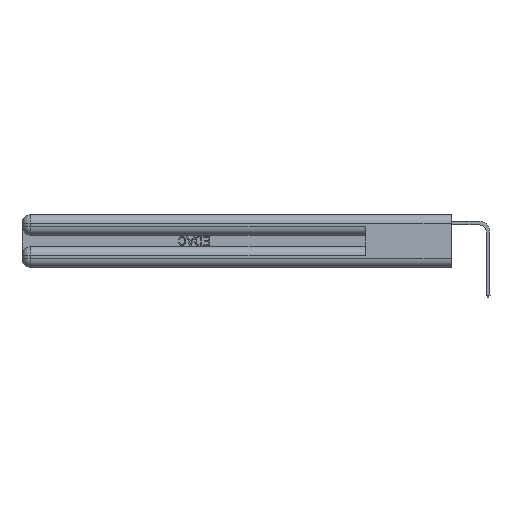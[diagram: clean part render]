
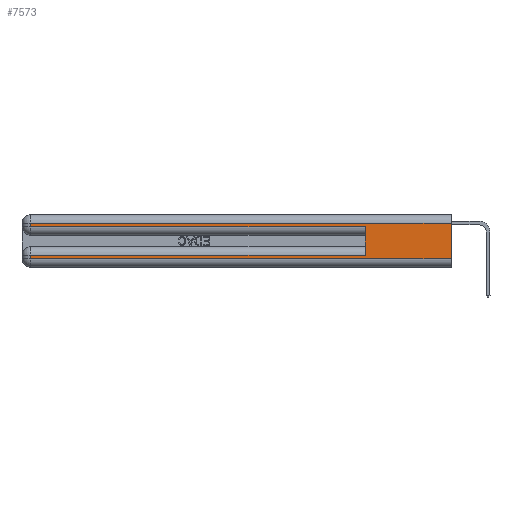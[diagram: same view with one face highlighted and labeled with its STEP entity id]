
A CAD part, left-side view. The second image highlights one B-rep face of the part: STEP entity #7573.
In plain terms, the highlighted planar face has unit normal (-1, 0, 0).
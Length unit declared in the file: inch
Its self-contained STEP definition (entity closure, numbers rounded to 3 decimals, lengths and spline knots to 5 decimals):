
#15 = VERTEX_POINT ( 'NONE', #14612 ) ;
#119 = CARTESIAN_POINT ( 'NONE',  ( 0., 0., 0.31 ) ) ;
#379 = VECTOR ( 'NONE', #6534, 39.37008 ) ;
#1182 = EDGE_CURVE ( 'NONE', #17346, #2728, #1530, .T. ) ;
#1530 = LINE ( 'NONE', #23896, #21152 ) ;
#1609 = LINE ( 'NONE', #19581, #3308 ) ;
#1701 = CARTESIAN_POINT ( 'NONE',  ( 0., 0.6, 0.285 ) ) ;
#2008 = LINE ( 'NONE', #19993, #13418 ) ;
#2155 = DIRECTION ( 'NONE',  ( 0., 1., 0. ) ) ;
#2191 = CARTESIAN_POINT ( 'NONE',  ( 0., 0., 0.37 ) ) ;
#2675 = CARTESIAN_POINT ( 'NONE',  ( 0., 2.94, 0.31 ) ) ;
#2728 = VERTEX_POINT ( 'NONE', #1701 ) ;
#3160 = ORIENTED_EDGE ( 'NONE', *, *, #20132, .T. ) ;
#3249 = CARTESIAN_POINT ( 'NONE',  ( 0., 0., 0.37 ) ) ;
#3308 = VECTOR ( 'NONE', #12978, 39.37008 ) ;
#3700 = CARTESIAN_POINT ( 'NONE',  ( 0., 0., 0.31 ) ) ;
#3762 = VERTEX_POINT ( 'NONE', #2675 ) ;
#5946 = VECTOR ( 'NONE', #15485, 39.37008 ) ;
#6268 = EDGE_CURVE ( 'NONE', #24456, #2728, #8498, .T. ) ;
#6534 = DIRECTION ( 'NONE',  ( 0., -1., 0. ) ) ;
#7437 = ORIENTED_EDGE ( 'NONE', *, *, #15135, .T. ) ;
#7573 = ADVANCED_FACE ( 'NONE', ( #27654 ), #14335, .F. ) ;
#8056 = DIRECTION ( 'NONE',  ( 0., -1., 0. ) ) ;
#8498 = LINE ( 'NONE', #26365, #9792 ) ;
#9051 = ORIENTED_EDGE ( 'NONE', *, *, #1182, .T. ) ;
#9096 = CARTESIAN_POINT ( 'NONE',  ( 0., 2.94, 0.085 ) ) ;
#9121 = ORIENTED_EDGE ( 'NONE', *, *, #6268, .F. ) ;
#9792 = VECTOR ( 'NONE', #15402, 39.37008 ) ;
#10291 = CARTESIAN_POINT ( 'NONE',  ( 0., 0.6, 0.085 ) ) ;
#10915 = VERTEX_POINT ( 'NONE', #119 ) ;
#11544 = DIRECTION ( 'NONE',  ( 0., 0., -1. ) ) ;
#11971 = CARTESIAN_POINT ( 'NONE',  ( 0., 2.94, 0.06 ) ) ;
#12207 = LINE ( 'NONE', #13982, #20094 ) ;
#12576 = EDGE_CURVE ( 'NONE', #24456, #14087, #2008, .T. ) ;
#12648 = ORIENTED_EDGE ( 'NONE', *, *, #12576, .T. ) ;
#12978 = DIRECTION ( 'NONE',  ( 0., 0., -1. ) ) ;
#13101 = LINE ( 'NONE', #28474, #379 ) ;
#13418 = VECTOR ( 'NONE', #2155, 39.37008 ) ;
#13982 = CARTESIAN_POINT ( 'NONE',  ( 0., 2.94, 0.37 ) ) ;
#14087 = VERTEX_POINT ( 'NONE', #9096 ) ;
#14335 = PLANE ( 'NONE',  #21048 ) ;
#14612 = CARTESIAN_POINT ( 'NONE',  ( 0., 0., 0.06 ) ) ;
#15135 = EDGE_CURVE ( 'NONE', #10915, #3762, #23746, .T. ) ;
#15200 = EDGE_LOOP ( 'NONE', ( #25194, #7437, #15966, #9051, #9121, #12648, #16920, #3160 ) ) ;
#15402 = DIRECTION ( 'NONE',  ( 0., 0., 1. ) ) ;
#15485 = DIRECTION ( 'NONE',  ( 0., 0., -1. ) ) ;
#15966 = ORIENTED_EDGE ( 'NONE', *, *, #27862, .T. ) ;
#16920 = ORIENTED_EDGE ( 'NONE', *, *, #27390, .T. ) ;
#17346 = VERTEX_POINT ( 'NONE', #19052 ) ;
#18420 = VERTEX_POINT ( 'NONE', #11971 ) ;
#18888 = VECTOR ( 'NONE', #19331, 39.37008 ) ;
#19052 = CARTESIAN_POINT ( 'NONE',  ( 0., 2.94, 0.285 ) ) ;
#19331 = DIRECTION ( 'NONE',  ( 0., 1., 0. ) ) ;
#19581 = CARTESIAN_POINT ( 'NONE',  ( 0., 2.94, 0.37 ) ) ;
#19820 = DIRECTION ( 'NONE',  ( 0., 0., -1. ) ) ;
#19993 = CARTESIAN_POINT ( 'NONE',  ( 0., 0., 0.085 ) ) ;
#20094 = VECTOR ( 'NONE', #19820, 39.37008 ) ;
#20132 = EDGE_CURVE ( 'NONE', #18420, #15, #13101, .T. ) ;
#20346 = DIRECTION ( 'NONE',  ( 1., 0., 0. ) ) ;
#21048 = AXIS2_PLACEMENT_3D ( 'NONE', #3249, #20346, #11544 ) ;
#21152 = VECTOR ( 'NONE', #8056, 39.37008 ) ;
#22603 = EDGE_CURVE ( 'NONE', #10915, #15, #28627, .T. ) ;
#23746 = LINE ( 'NONE', #3700, #18888 ) ;
#23896 = CARTESIAN_POINT ( 'NONE',  ( 0., 0., 0.285 ) ) ;
#24456 = VERTEX_POINT ( 'NONE', #10291 ) ;
#25194 = ORIENTED_EDGE ( 'NONE', *, *, #22603, .F. ) ;
#26365 = CARTESIAN_POINT ( 'NONE',  ( 0., 0.6, 0.145 ) ) ;
#27390 = EDGE_CURVE ( 'NONE', #14087, #18420, #1609, .T. ) ;
#27654 = FACE_OUTER_BOUND ( 'NONE', #15200, .T. ) ;
#27862 = EDGE_CURVE ( 'NONE', #3762, #17346, #12207, .T. ) ;
#28474 = CARTESIAN_POINT ( 'NONE',  ( 0., 0., 0.06 ) ) ;
#28627 = LINE ( 'NONE', #2191, #5946 ) ;
